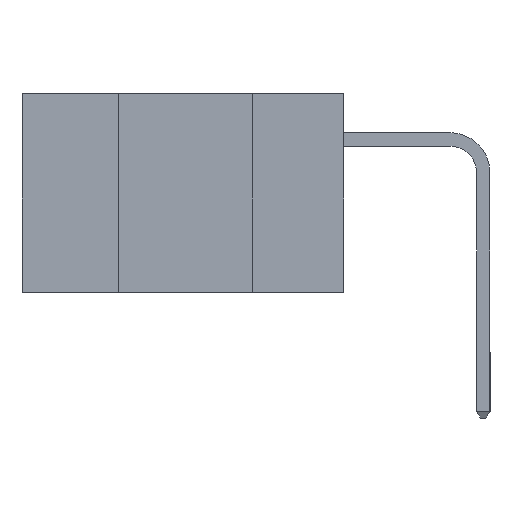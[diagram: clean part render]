
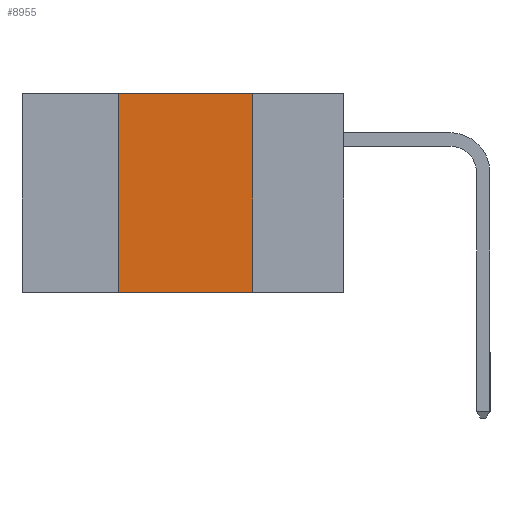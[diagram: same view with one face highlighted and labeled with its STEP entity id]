
A CAD part, left-side view. The second image highlights one B-rep face of the part: STEP entity #8955.
In plain terms, the highlighted planar face has unit normal (-1, 0, 0).
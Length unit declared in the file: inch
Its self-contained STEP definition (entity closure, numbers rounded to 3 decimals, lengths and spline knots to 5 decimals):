
#1338 = VECTOR ( 'NONE', #16247, 39.37008 ) ;
#1681 = ORIENTED_EDGE ( 'NONE', *, *, #3112, .F. ) ;
#3112 = EDGE_CURVE ( 'NONE', #14191, #23400, #12749, .T. ) ;
#4777 = VECTOR ( 'NONE', #17366, 39.37008 ) ;
#5225 = FACE_OUTER_BOUND ( 'NONE', #26847, .T. ) ;
#5589 = DIRECTION ( 'NONE',  ( 1., 0., 0. ) ) ;
#6592 = VECTOR ( 'NONE', #7578, 39.37008 ) ;
#7177 = EDGE_CURVE ( 'NONE', #13100, #23400, #20010, .T. ) ;
#7552 = AXIS2_PLACEMENT_3D ( 'NONE', #15967, #5589, #17872 ) ;
#7578 = DIRECTION ( 'NONE',  ( 0., -1., 0. ) ) ;
#7596 = CARTESIAN_POINT ( 'NONE',  ( 0., 0.42, 0. ) ) ;
#7752 = CARTESIAN_POINT ( 'NONE',  ( 0., 0.17, 0. ) ) ;
#8955 = ADVANCED_FACE ( 'NONE', ( #5225 ), #9430, .F. ) ;
#9430 = PLANE ( 'NONE',  #7552 ) ;
#10625 = CARTESIAN_POINT ( 'NONE',  ( 0., 0.17, -0.37 ) ) ;
#11256 = EDGE_CURVE ( 'NONE', #19280, #14191, #16287, .T. ) ;
#11568 = CARTESIAN_POINT ( 'NONE',  ( 0., 0.42, 0. ) ) ;
#12749 = LINE ( 'NONE', #15255, #15354 ) ;
#13100 = VERTEX_POINT ( 'NONE', #13641 ) ;
#13641 = CARTESIAN_POINT ( 'NONE',  ( 0., 0.42, -0.37 ) ) ;
#14191 = VERTEX_POINT ( 'NONE', #7752 ) ;
#14468 = ORIENTED_EDGE ( 'NONE', *, *, #7177, .T. ) ;
#15255 = CARTESIAN_POINT ( 'NONE',  ( 0., 0.17, 0. ) ) ;
#15277 = CARTESIAN_POINT ( 'NONE',  ( 0., 0.6, 0. ) ) ;
#15354 = VECTOR ( 'NONE', #21197, 39.37008 ) ;
#15468 = LINE ( 'NONE', #7596, #1338 ) ;
#15967 = CARTESIAN_POINT ( 'NONE',  ( 0., 0.6, 0. ) ) ;
#16247 = DIRECTION ( 'NONE',  ( 0., 0., 1. ) ) ;
#16287 = LINE ( 'NONE', #15277, #4777 ) ;
#17366 = DIRECTION ( 'NONE',  ( 0., -1., 0. ) ) ;
#17872 = DIRECTION ( 'NONE',  ( 0., 0., -1. ) ) ;
#18688 = EDGE_CURVE ( 'NONE', #13100, #19280, #15468, .T. ) ;
#19280 = VERTEX_POINT ( 'NONE', #11568 ) ;
#20010 = LINE ( 'NONE', #22315, #6592 ) ;
#20040 = ORIENTED_EDGE ( 'NONE', *, *, #18688, .F. ) ;
#21197 = DIRECTION ( 'NONE',  ( 0., 0., -1. ) ) ;
#22315 = CARTESIAN_POINT ( 'NONE',  ( 0., 0.6, -0.37 ) ) ;
#23400 = VERTEX_POINT ( 'NONE', #10625 ) ;
#25642 = ORIENTED_EDGE ( 'NONE', *, *, #11256, .F. ) ;
#26847 = EDGE_LOOP ( 'NONE', ( #1681, #25642, #20040, #14468 ) ) ;
